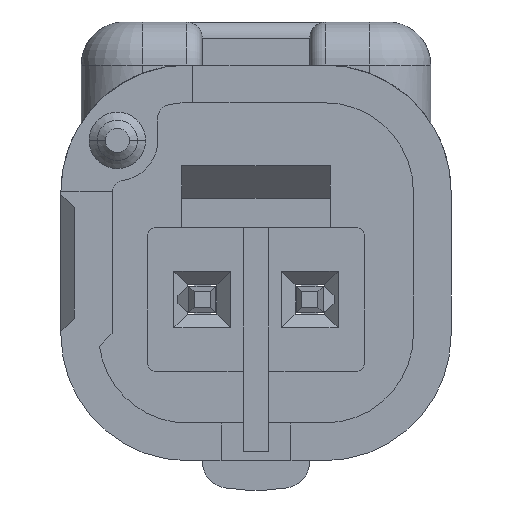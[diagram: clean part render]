
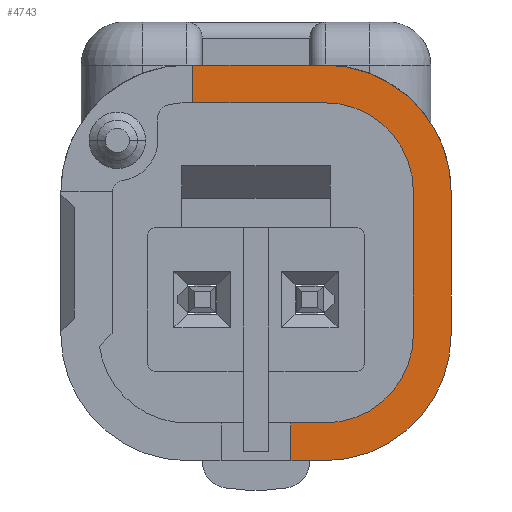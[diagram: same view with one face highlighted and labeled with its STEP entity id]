
A CAD part, front view. The second image highlights one B-rep face of the part: STEP entity #4743.
In plain terms, the highlighted face is planar.
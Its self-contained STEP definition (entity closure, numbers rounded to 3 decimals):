
#127 = CARTESIAN_POINT ( 'NONE',  ( 7.6, 1.325, -1.275 ) ) ;
#225 = CIRCLE ( 'NONE', #10345, 2.35 ) ;
#693 = LINE ( 'NONE', #8127, #5674 ) ;
#810 = CARTESIAN_POINT ( 'NONE',  ( 7.6, 2.975, -1.275 ) ) ;
#1298 = VERTEX_POINT ( 'NONE', #8820 ) ;
#1587 = PLANE ( 'NONE',  #11118 ) ;
#1594 = EDGE_LOOP ( 'NONE', ( #8796, #3757, #14410, #7467, #9056, #5828, #3635, #12567, #2030, #6021, #3765, #13296 ) ) ;
#1943 = CARTESIAN_POINT ( 'NONE',  ( 7.6, -1.325, -1.275 ) ) ;
#2030 = ORIENTED_EDGE ( 'NONE', *, *, #4216, .T. ) ;
#2358 = CIRCLE ( 'NONE', #6906, 2.35 ) ;
#2408 = LINE ( 'NONE', #14466, #12790 ) ;
#2472 = CARTESIAN_POINT ( 'NONE',  ( 7.6, 3.675, 1.275 ) ) ;
#2616 = CARTESIAN_POINT ( 'NONE',  ( 7.6, 1.325, -3.625 ) ) ;
#3175 = VERTEX_POINT ( 'NONE', #4813 ) ;
#3635 = ORIENTED_EDGE ( 'NONE', *, *, #15278, .F. ) ;
#3757 = ORIENTED_EDGE ( 'NONE', *, *, #15528, .F. ) ;
#3765 = ORIENTED_EDGE ( 'NONE', *, *, #12250, .T. ) ;
#3993 = CARTESIAN_POINT ( 'NONE',  ( 7.6, 1.325, -1.275 ) ) ;
#4216 = EDGE_CURVE ( 'NONE', #4287, #13574, #225, .T. ) ;
#4287 = VERTEX_POINT ( 'NONE', #6520 ) ;
#4339 = DIRECTION ( 'NONE',  ( 0., 1., 0. ) ) ;
#4686 = EDGE_CURVE ( 'NONE', #7332, #3175, #9987, .T. ) ;
#4743 = ADVANCED_FACE ( 'NONE', ( #15144 ), #1587, .T. ) ;
#4813 = CARTESIAN_POINT ( 'NONE',  ( 7.6, 3.675, 1.175 ) ) ;
#4925 = VECTOR ( 'NONE', #11502, 1000. ) ;
#5002 = EDGE_CURVE ( 'NONE', #9957, #6907, #11130, .T. ) ;
#5372 = DIRECTION ( 'NONE',  ( 1., 0., 0. ) ) ;
#5376 = AXIS2_PLACEMENT_3D ( 'NONE', #3993, #7624, #10097 ) ;
#5674 = VECTOR ( 'NONE', #5830, 1000. ) ;
#5747 = EDGE_CURVE ( 'NONE', #12266, #3175, #9156, .T. ) ;
#5800 = LINE ( 'NONE', #810, #15580 ) ;
#5828 = ORIENTED_EDGE ( 'NONE', *, *, #12176, .F. ) ;
#5830 = DIRECTION ( 'NONE',  ( 0., 1., 0. ) ) ;
#5982 = CARTESIAN_POINT ( 'NONE',  ( 7.6, -2.975, -0.65 ) ) ;
#6021 = ORIENTED_EDGE ( 'NONE', *, *, #13373, .T. ) ;
#6193 = CARTESIAN_POINT ( 'NONE',  ( 7.6, -2.975, -1.275 ) ) ;
#6264 = DIRECTION ( 'NONE',  ( 0., 0., 1. ) ) ;
#6520 = CARTESIAN_POINT ( 'NONE',  ( 7.6, -3.675, -1.275 ) ) ;
#6631 = VERTEX_POINT ( 'NONE', #10774 ) ;
#6906 = AXIS2_PLACEMENT_3D ( 'NONE', #127, #13289, #12026 ) ;
#6907 = VERTEX_POINT ( 'NONE', #10203 ) ;
#7254 = CARTESIAN_POINT ( 'NONE',  ( 7.6, 2.975, 1.175 ) ) ;
#7275 = EDGE_CURVE ( 'NONE', #6631, #1298, #12754, .T. ) ;
#7321 = AXIS2_PLACEMENT_3D ( 'NONE', #1943, #8031, #13040 ) ;
#7332 = VERTEX_POINT ( 'NONE', #15324 ) ;
#7387 = DIRECTION ( 'NONE',  ( 0., 1., 0. ) ) ;
#7467 = ORIENTED_EDGE ( 'NONE', *, *, #14659, .F. ) ;
#7620 = DIRECTION ( 'NONE',  ( 1., 0., 0. ) ) ;
#7624 = DIRECTION ( 'NONE',  ( 1., 0., 0. ) ) ;
#7760 = CARTESIAN_POINT ( 'NONE',  ( 7.6, -3.675, 1.275 ) ) ;
#7833 = DIRECTION ( 'NONE',  ( 0., 1., 0. ) ) ;
#8031 = DIRECTION ( 'NONE',  ( 1., 0., 0. ) ) ;
#8067 = CARTESIAN_POINT ( 'NONE',  ( 7.6, -1.325, -2.925 ) ) ;
#8127 = CARTESIAN_POINT ( 'NONE',  ( 7.6, 1.325, -3.625 ) ) ;
#8752 = CARTESIAN_POINT ( 'NONE',  ( 7.6, -1.325, -1.275 ) ) ;
#8796 = ORIENTED_EDGE ( 'NONE', *, *, #5747, .F. ) ;
#8820 = CARTESIAN_POINT ( 'NONE',  ( 7.6, 2.975, -1.275 ) ) ;
#8839 = VECTOR ( 'NONE', #6264, 1000. ) ;
#8964 = EDGE_CURVE ( 'NONE', #9124, #4287, #13953, .T. ) ;
#9056 = ORIENTED_EDGE ( 'NONE', *, *, #5002, .F. ) ;
#9105 = LINE ( 'NONE', #8067, #12272 ) ;
#9124 = VERTEX_POINT ( 'NONE', #9405 ) ;
#9156 = LINE ( 'NONE', #12897, #9368 ) ;
#9165 = DIRECTION ( 'NONE',  ( 0., 0., -1. ) ) ;
#9368 = VECTOR ( 'NONE', #14000, 1000. ) ;
#9405 = CARTESIAN_POINT ( 'NONE',  ( 7.6, -3.675, -0.65 ) ) ;
#9957 = VERTEX_POINT ( 'NONE', #6193 ) ;
#9987 = LINE ( 'NONE', #2472, #8839 ) ;
#10097 = DIRECTION ( 'NONE',  ( 0., 0., -1. ) ) ;
#10203 = CARTESIAN_POINT ( 'NONE',  ( 7.6, -1.325, -2.925 ) ) ;
#10345 = AXIS2_PLACEMENT_3D ( 'NONE', #8752, #7620, #12481 ) ;
#10774 = CARTESIAN_POINT ( 'NONE',  ( 7.6, 1.325, -2.925 ) ) ;
#11118 = AXIS2_PLACEMENT_3D ( 'NONE', #15068, #5372, #7833 ) ;
#11130 = CIRCLE ( 'NONE', #7321, 1.65 ) ;
#11502 = DIRECTION ( 'NONE',  ( 0., 0., -1. ) ) ;
#11733 = VECTOR ( 'NONE', #9165, 1000. ) ;
#12026 = DIRECTION ( 'NONE',  ( 0., 0., -1. ) ) ;
#12176 = EDGE_CURVE ( 'NONE', #15255, #9957, #14088, .T. ) ;
#12250 = EDGE_CURVE ( 'NONE', #14628, #7332, #2358, .T. ) ;
#12266 = VERTEX_POINT ( 'NONE', #7254 ) ;
#12272 = VECTOR ( 'NONE', #4339, 1000. ) ;
#12481 = DIRECTION ( 'NONE',  ( 0., 0., -1. ) ) ;
#12567 = ORIENTED_EDGE ( 'NONE', *, *, #8964, .T. ) ;
#12754 = CIRCLE ( 'NONE', #5376, 1.65 ) ;
#12790 = VECTOR ( 'NONE', #7387, 1000. ) ;
#12793 = DIRECTION ( 'NONE',  ( 0., 0., 1. ) ) ;
#12897 = CARTESIAN_POINT ( 'NONE',  ( 7.6, 3.675, 1.175 ) ) ;
#13040 = DIRECTION ( 'NONE',  ( 0., 0., -1. ) ) ;
#13289 = DIRECTION ( 'NONE',  ( 1., 0., 0. ) ) ;
#13296 = ORIENTED_EDGE ( 'NONE', *, *, #4686, .T. ) ;
#13373 = EDGE_CURVE ( 'NONE', #13574, #14628, #693, .T. ) ;
#13574 = VERTEX_POINT ( 'NONE', #14482 ) ;
#13953 = LINE ( 'NONE', #7760, #4925 ) ;
#14000 = DIRECTION ( 'NONE',  ( 0., 1., 0. ) ) ;
#14088 = LINE ( 'NONE', #14240, #11733 ) ;
#14240 = CARTESIAN_POINT ( 'NONE',  ( 7.6, -2.975, 1.275 ) ) ;
#14410 = ORIENTED_EDGE ( 'NONE', *, *, #7275, .F. ) ;
#14466 = CARTESIAN_POINT ( 'NONE',  ( 7.6, -1.325, -0.65 ) ) ;
#14482 = CARTESIAN_POINT ( 'NONE',  ( 7.6, -1.325, -3.625 ) ) ;
#14628 = VERTEX_POINT ( 'NONE', #2616 ) ;
#14659 = EDGE_CURVE ( 'NONE', #6907, #6631, #9105, .T. ) ;
#15068 = CARTESIAN_POINT ( 'NONE',  ( 7.6, -1.325, 1.275 ) ) ;
#15144 = FACE_OUTER_BOUND ( 'NONE', #1594, .T. ) ;
#15255 = VERTEX_POINT ( 'NONE', #5982 ) ;
#15278 = EDGE_CURVE ( 'NONE', #9124, #15255, #2408, .T. ) ;
#15324 = CARTESIAN_POINT ( 'NONE',  ( 7.6, 3.675, -1.275 ) ) ;
#15528 = EDGE_CURVE ( 'NONE', #1298, #12266, #5800, .T. ) ;
#15580 = VECTOR ( 'NONE', #12793, 1000. ) ;
